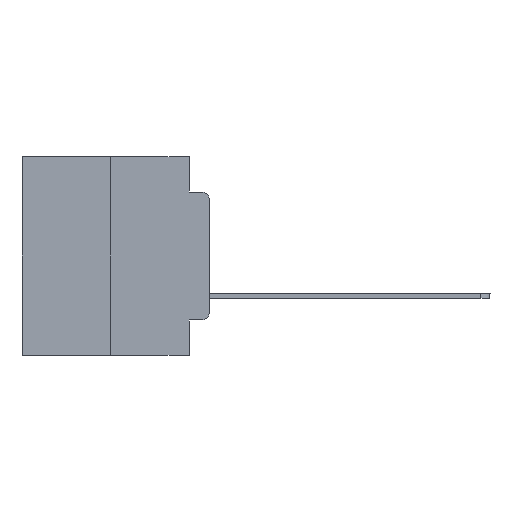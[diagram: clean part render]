
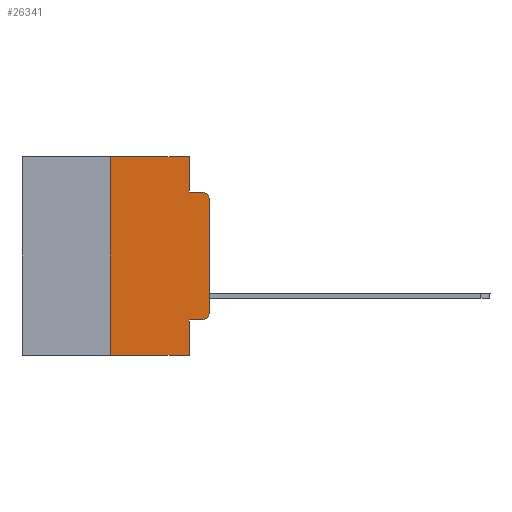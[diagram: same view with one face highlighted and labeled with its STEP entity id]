
A CAD part, left-side view. The second image highlights one B-rep face of the part: STEP entity #26341.
In plain terms, the highlighted planar face has unit normal (-1, 0, 0).
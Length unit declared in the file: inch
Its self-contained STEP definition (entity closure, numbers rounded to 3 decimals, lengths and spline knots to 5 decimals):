
#702 = VECTOR ( 'NONE', #16008, 39.37008 ) ;
#1220 = DIRECTION ( 'NONE',  ( -1., 0., 0. ) ) ;
#1506 = LINE ( 'NONE', #22742, #7228 ) ;
#1583 = CARTESIAN_POINT ( 'NONE',  ( 0., 0., -0.1085 ) ) ;
#1609 = EDGE_CURVE ( 'NONE', #12583, #13169, #9133, .T. ) ;
#1726 = CARTESIAN_POINT ( 'NONE',  ( 0., 0.051, -0.4115 ) ) ;
#1848 = VECTOR ( 'NONE', #15848, 39.37008 ) ;
#1906 = AXIS2_PLACEMENT_3D ( 'NONE', #2699, #18221, #22123 ) ;
#2002 = ORIENTED_EDGE ( 'NONE', *, *, #15819, .T. ) ;
#2144 = VERTEX_POINT ( 'NONE', #20277 ) ;
#2366 = DIRECTION ( 'NONE',  ( 0., -1., 0. ) ) ;
#2414 = VECTOR ( 'NONE', #7065, 39.37008 ) ;
#2699 = CARTESIAN_POINT ( 'NONE',  ( 0., 0.473, 0. ) ) ;
#2780 = ORIENTED_EDGE ( 'NONE', *, *, #8788, .F. ) ;
#2884 = VERTEX_POINT ( 'NONE', #4697 ) ;
#2991 = ORIENTED_EDGE ( 'NONE', *, *, #9024, .F. ) ;
#3558 = VERTEX_POINT ( 'NONE', #25394 ) ;
#3669 = DIRECTION ( 'NONE',  ( 0., -1., 0. ) ) ;
#3837 = VECTOR ( 'NONE', #3669, 39.37008 ) ;
#4697 = CARTESIAN_POINT ( 'NONE',  ( 0., 0.25, 0. ) ) ;
#4751 = EDGE_CURVE ( 'NONE', #16943, #13169, #7694, .T. ) ;
#4969 = VERTEX_POINT ( 'NONE', #11170 ) ;
#5351 = CIRCLE ( 'NONE', #7161, 0.02 ) ;
#5745 = VECTOR ( 'NONE', #19905, 39.37008 ) ;
#5779 = CIRCLE ( 'NONE', #24090, 0.02 ) ;
#6279 = DIRECTION ( 'NONE',  ( -1., 0., 0. ) ) ;
#7065 = DIRECTION ( 'NONE',  ( 0., -1., 0. ) ) ;
#7161 = AXIS2_PLACEMENT_3D ( 'NONE', #8383, #6279, #19148 ) ;
#7228 = VECTOR ( 'NONE', #7935, 39.37008 ) ;
#7587 = LINE ( 'NONE', #16896, #702 ) ;
#7694 = LINE ( 'NONE', #27096, #9019 ) ;
#7935 = DIRECTION ( 'NONE',  ( 0., 0., 1. ) ) ;
#8383 = CARTESIAN_POINT ( 'NONE',  ( 0., 0.02, -0.3915 ) ) ;
#8788 = EDGE_CURVE ( 'NONE', #2884, #20588, #17192, .T. ) ;
#9019 = VECTOR ( 'NONE', #9921, 39.37008 ) ;
#9024 = EDGE_CURVE ( 'NONE', #12583, #2884, #1506, .T. ) ;
#9133 = LINE ( 'NONE', #21712, #5745 ) ;
#9136 = FACE_OUTER_BOUND ( 'NONE', #23613, .T. ) ;
#9794 = LINE ( 'NONE', #11764, #1848 ) ;
#9921 = DIRECTION ( 'NONE',  ( 0., 0., -1. ) ) ;
#11127 = CARTESIAN_POINT ( 'NONE',  ( 0., 0.051, -0.0885 ) ) ;
#11170 = CARTESIAN_POINT ( 'NONE',  ( 0., 0.02, -0.4115 ) ) ;
#11692 = VERTEX_POINT ( 'NONE', #14276 ) ;
#11764 = CARTESIAN_POINT ( 'NONE',  ( 0., 0.051, 0. ) ) ;
#12583 = VERTEX_POINT ( 'NONE', #25876 ) ;
#13169 = VERTEX_POINT ( 'NONE', #22085 ) ;
#14276 = CARTESIAN_POINT ( 'NONE',  ( 0., 0.051, -0.0885 ) ) ;
#15198 = EDGE_CURVE ( 'NONE', #11692, #3558, #19656, .T. ) ;
#15819 = EDGE_CURVE ( 'NONE', #2144, #26103, #7587, .T. ) ;
#15848 = DIRECTION ( 'NONE',  ( 0., 0., -1. ) ) ;
#16008 = DIRECTION ( 'NONE',  ( 0., 0., 1. ) ) ;
#16643 = CARTESIAN_POINT ( 'NONE',  ( 0., 0.051, 0. ) ) ;
#16896 = CARTESIAN_POINT ( 'NONE',  ( 0., 0., 0. ) ) ;
#16943 = VERTEX_POINT ( 'NONE', #1726 ) ;
#17192 = LINE ( 'NONE', #19133, #19734 ) ;
#18221 = DIRECTION ( 'NONE',  ( 1., 0., 0. ) ) ;
#18271 = CARTESIAN_POINT ( 'NONE',  ( 0., 0.02, -0.1085 ) ) ;
#18440 = ORIENTED_EDGE ( 'NONE', *, *, #4751, .F. ) ;
#18617 = EDGE_CURVE ( 'NONE', #16943, #4969, #20341, .T. ) ;
#19133 = CARTESIAN_POINT ( 'NONE',  ( 0., 0.473, 0. ) ) ;
#19148 = DIRECTION ( 'NONE',  ( 0., 0., -1. ) ) ;
#19656 = LINE ( 'NONE', #11127, #2414 ) ;
#19734 = VECTOR ( 'NONE', #2366, 39.37008 ) ;
#19905 = DIRECTION ( 'NONE',  ( 0., -1., 0. ) ) ;
#20049 = EDGE_CURVE ( 'NONE', #26103, #3558, #5779, .T. ) ;
#20245 = ORIENTED_EDGE ( 'NONE', *, *, #20478, .T. ) ;
#20277 = CARTESIAN_POINT ( 'NONE',  ( 0., 0., -0.3915 ) ) ;
#20341 = LINE ( 'NONE', #22416, #3837 ) ;
#20478 = EDGE_CURVE ( 'NONE', #4969, #2144, #5351, .T. ) ;
#20588 = VERTEX_POINT ( 'NONE', #16643 ) ;
#20907 = ORIENTED_EDGE ( 'NONE', *, *, #20049, .T. ) ;
#21675 = ORIENTED_EDGE ( 'NONE', *, *, #23535, .F. ) ;
#21712 = CARTESIAN_POINT ( 'NONE',  ( 0., 0.473, -0.5 ) ) ;
#22085 = CARTESIAN_POINT ( 'NONE',  ( 0., 0.051, -0.5 ) ) ;
#22123 = DIRECTION ( 'NONE',  ( 0., 0., -1. ) ) ;
#22416 = CARTESIAN_POINT ( 'NONE',  ( 0., 0.051, -0.4115 ) ) ;
#22600 = ORIENTED_EDGE ( 'NONE', *, *, #1609, .T. ) ;
#22621 = ORIENTED_EDGE ( 'NONE', *, *, #15198, .F. ) ;
#22742 = CARTESIAN_POINT ( 'NONE',  ( 0., 0.25, 0. ) ) ;
#23535 = EDGE_CURVE ( 'NONE', #20588, #11692, #9794, .T. ) ;
#23613 = EDGE_LOOP ( 'NONE', ( #2002, #20907, #22621, #21675, #2780, #2991, #22600, #18440, #26268, #20245 ) ) ;
#24090 = AXIS2_PLACEMENT_3D ( 'NONE', #18271, #1220, #26772 ) ;
#25394 = CARTESIAN_POINT ( 'NONE',  ( 0., 0.02, -0.0885 ) ) ;
#25876 = CARTESIAN_POINT ( 'NONE',  ( 0., 0.25, -0.5 ) ) ;
#26103 = VERTEX_POINT ( 'NONE', #1583 ) ;
#26268 = ORIENTED_EDGE ( 'NONE', *, *, #18617, .T. ) ;
#26341 = ADVANCED_FACE ( 'NONE', ( #9136 ), #26592, .F. ) ;
#26592 = PLANE ( 'NONE',  #1906 ) ;
#26772 = DIRECTION ( 'NONE',  ( 0., 0., -1. ) ) ;
#27096 = CARTESIAN_POINT ( 'NONE',  ( 0., 0.051, 0. ) ) ;
